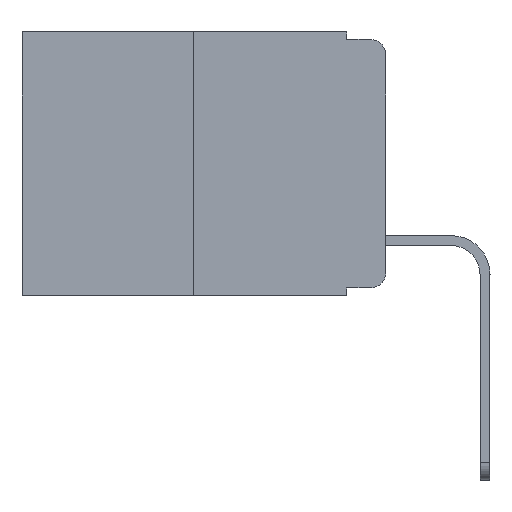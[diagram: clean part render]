
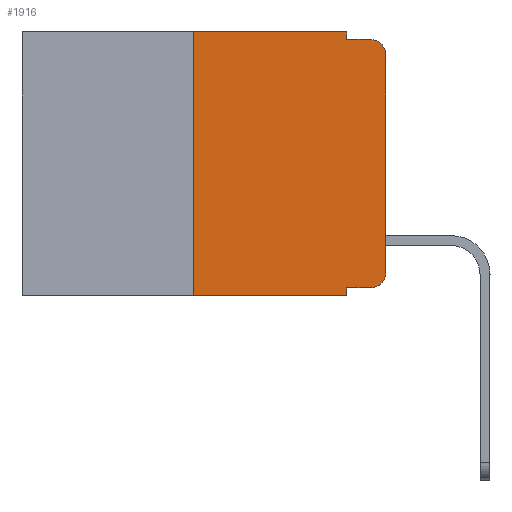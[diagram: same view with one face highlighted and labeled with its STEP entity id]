
A CAD part, left-side view. The second image highlights one B-rep face of the part: STEP entity #1916.
In plain terms, the highlighted planar face has unit normal (-1, 0, 0).
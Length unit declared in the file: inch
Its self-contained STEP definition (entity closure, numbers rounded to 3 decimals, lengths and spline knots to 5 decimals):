
#243 = CARTESIAN_POINT ( 'NONE',  ( 0., 0.051, -0.343 ) ) ;
#392 = CARTESIAN_POINT ( 'NONE',  ( 0., 0.02, -0.313 ) ) ;
#397 = VERTEX_POINT ( 'NONE', #6595 ) ;
#946 = DIRECTION ( 'NONE',  ( 0., 0., -1. ) ) ;
#976 = CIRCLE ( 'NONE', #5973, 0.02 ) ;
#1004 = CARTESIAN_POINT ( 'NONE',  ( 0., 0., -0.313 ) ) ;
#1026 = CARTESIAN_POINT ( 'NONE',  ( 0., 0., 0. ) ) ;
#1071 = VECTOR ( 'NONE', #9937, 39.37008 ) ;
#1166 = VERTEX_POINT ( 'NONE', #8238 ) ;
#1252 = LINE ( 'NONE', #12166, #1071 ) ;
#1272 = VECTOR ( 'NONE', #5008, 39.37008 ) ;
#1299 = LINE ( 'NONE', #11372, #3613 ) ;
#1374 = DIRECTION ( 'NONE',  ( 0., 0., 1. ) ) ;
#1647 = LINE ( 'NONE', #11631, #6978 ) ;
#1744 = ORIENTED_EDGE ( 'NONE', *, *, #3170, .T. ) ;
#1916 = ADVANCED_FACE ( 'NONE', ( #7012 ), #5526, .F. ) ;
#2010 = VECTOR ( 'NONE', #3751, 39.37008 ) ;
#2164 = LINE ( 'NONE', #1026, #13307 ) ;
#2355 = LINE ( 'NONE', #4869, #2010 ) ;
#2381 = CARTESIAN_POINT ( 'NONE',  ( 0., 0.02, -0.01 ) ) ;
#2397 = DIRECTION ( 'NONE',  ( -1., 0., 0. ) ) ;
#2746 = VERTEX_POINT ( 'NONE', #243 ) ;
#2749 = VERTEX_POINT ( 'NONE', #10655 ) ;
#2755 = EDGE_CURVE ( 'NONE', #3452, #397, #2164, .T. ) ;
#2881 = DIRECTION ( 'NONE',  ( 0., -1., 0. ) ) ;
#3170 = EDGE_CURVE ( 'NONE', #12827, #3452, #976, .T. ) ;
#3452 = VERTEX_POINT ( 'NONE', #1004 ) ;
#3575 = VECTOR ( 'NONE', #946, 39.37008 ) ;
#3613 = VECTOR ( 'NONE', #2881, 39.37008 ) ;
#3751 = DIRECTION ( 'NONE',  ( 0., -1., 0. ) ) ;
#3966 = CARTESIAN_POINT ( 'NONE',  ( 0., 0.051, 0. ) ) ;
#3979 = EDGE_CURVE ( 'NONE', #7098, #12827, #1647, .T. ) ;
#4250 = LINE ( 'NONE', #3966, #3575 ) ;
#4375 = AXIS2_PLACEMENT_3D ( 'NONE', #13708, #7427, #8484 ) ;
#4522 = EDGE_CURVE ( 'NONE', #2749, #6326, #1299, .T. ) ;
#4538 = CARTESIAN_POINT ( 'NONE',  ( 0., 0.25, 0. ) ) ;
#4576 = CARTESIAN_POINT ( 'NONE',  ( 0., 0.02, -0.03 ) ) ;
#4869 = CARTESIAN_POINT ( 'NONE',  ( 0., 0.473, -0.343 ) ) ;
#5008 = DIRECTION ( 'NONE',  ( 0., -1., 0. ) ) ;
#5079 = VERTEX_POINT ( 'NONE', #11358 ) ;
#5277 = EDGE_CURVE ( 'NONE', #1166, #13309, #8742, .T. ) ;
#5334 = DIRECTION ( 'NONE',  ( 0., -1., 0. ) ) ;
#5526 = PLANE ( 'NONE',  #4375 ) ;
#5742 = DIRECTION ( 'NONE',  ( 0., 0., -1. ) ) ;
#5779 = CARTESIAN_POINT ( 'NONE',  ( 0., 0.051, -0.333 ) ) ;
#5973 = AXIS2_PLACEMENT_3D ( 'NONE', #392, #7749, #5742 ) ;
#6326 = VERTEX_POINT ( 'NONE', #2381 ) ;
#6595 = CARTESIAN_POINT ( 'NONE',  ( 0., 0., -0.03 ) ) ;
#6749 = ORIENTED_EDGE ( 'NONE', *, *, #4522, .F. ) ;
#6978 = VECTOR ( 'NONE', #5334, 39.37008 ) ;
#7012 = FACE_OUTER_BOUND ( 'NONE', #9054, .T. ) ;
#7098 = VERTEX_POINT ( 'NONE', #5779 ) ;
#7427 = DIRECTION ( 'NONE',  ( 1., 0., 0. ) ) ;
#7650 = DIRECTION ( 'NONE',  ( 0., 0., -1. ) ) ;
#7749 = DIRECTION ( 'NONE',  ( -1., 0., 0. ) ) ;
#8080 = CIRCLE ( 'NONE', #11341, 0.02 ) ;
#8176 = ORIENTED_EDGE ( 'NONE', *, *, #12012, .F. ) ;
#8238 = CARTESIAN_POINT ( 'NONE',  ( 0., 0.25, 0. ) ) ;
#8484 = DIRECTION ( 'NONE',  ( 0., 0., -1. ) ) ;
#8742 = LINE ( 'NONE', #11340, #1272 ) ;
#8753 = ORIENTED_EDGE ( 'NONE', *, *, #12771, .T. ) ;
#8802 = ORIENTED_EDGE ( 'NONE', *, *, #2755, .T. ) ;
#9054 = EDGE_LOOP ( 'NONE', ( #8802, #11566, #6749, #13214, #11469, #8176, #8753, #12595, #12448, #1744 ) ) ;
#9648 = EDGE_CURVE ( 'NONE', #13309, #2749, #4250, .T. ) ;
#9905 = EDGE_CURVE ( 'NONE', #397, #6326, #8080, .T. ) ;
#9937 = DIRECTION ( 'NONE',  ( 0., 0., -1. ) ) ;
#10073 = EDGE_CURVE ( 'NONE', #7098, #2746, #1252, .T. ) ;
#10655 = CARTESIAN_POINT ( 'NONE',  ( 0., 0.051, -0.01 ) ) ;
#10989 = DIRECTION ( 'NONE',  ( 0., 0., 1. ) ) ;
#11142 = CARTESIAN_POINT ( 'NONE',  ( 0., 0.051, 0. ) ) ;
#11161 = LINE ( 'NONE', #4538, #12832 ) ;
#11340 = CARTESIAN_POINT ( 'NONE',  ( 0., 0.473, 0. ) ) ;
#11341 = AXIS2_PLACEMENT_3D ( 'NONE', #4576, #2397, #7650 ) ;
#11358 = CARTESIAN_POINT ( 'NONE',  ( 0., 0.25, -0.343 ) ) ;
#11372 = CARTESIAN_POINT ( 'NONE',  ( 0., 0.051, -0.01 ) ) ;
#11469 = ORIENTED_EDGE ( 'NONE', *, *, #5277, .F. ) ;
#11566 = ORIENTED_EDGE ( 'NONE', *, *, #9905, .T. ) ;
#11631 = CARTESIAN_POINT ( 'NONE',  ( 0., 0.051, -0.333 ) ) ;
#12012 = EDGE_CURVE ( 'NONE', #5079, #1166, #11161, .T. ) ;
#12166 = CARTESIAN_POINT ( 'NONE',  ( 0., 0.051, 0. ) ) ;
#12448 = ORIENTED_EDGE ( 'NONE', *, *, #3979, .T. ) ;
#12595 = ORIENTED_EDGE ( 'NONE', *, *, #10073, .F. ) ;
#12771 = EDGE_CURVE ( 'NONE', #5079, #2746, #2355, .T. ) ;
#12827 = VERTEX_POINT ( 'NONE', #13388 ) ;
#12832 = VECTOR ( 'NONE', #1374, 39.37008 ) ;
#13214 = ORIENTED_EDGE ( 'NONE', *, *, #9648, .F. ) ;
#13307 = VECTOR ( 'NONE', #10989, 39.37008 ) ;
#13309 = VERTEX_POINT ( 'NONE', #11142 ) ;
#13388 = CARTESIAN_POINT ( 'NONE',  ( 0., 0.02, -0.333 ) ) ;
#13708 = CARTESIAN_POINT ( 'NONE',  ( 0., 0.473, 0. ) ) ;
